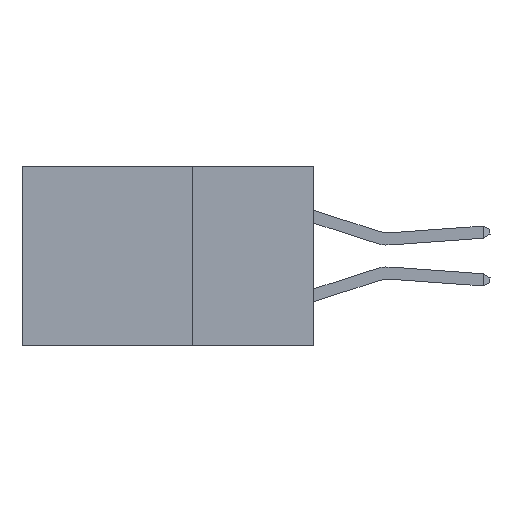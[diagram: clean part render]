
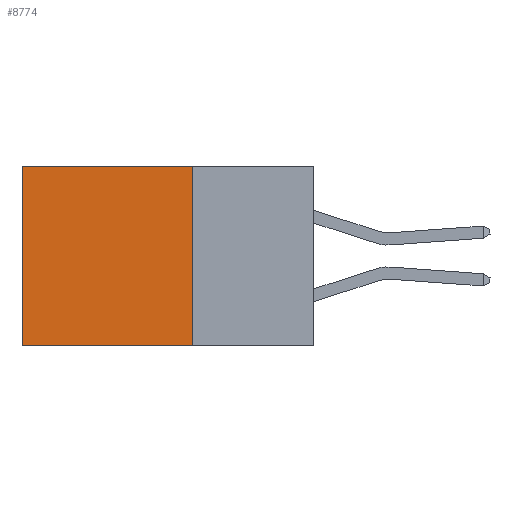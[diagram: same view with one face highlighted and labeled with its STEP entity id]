
A CAD part, left-side view. The second image highlights one B-rep face of the part: STEP entity #8774.
In plain terms, the highlighted planar face has unit normal (-1, 0, 0).
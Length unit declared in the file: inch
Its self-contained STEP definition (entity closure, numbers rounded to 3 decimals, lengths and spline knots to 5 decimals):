
#2572 = VERTEX_POINT ( 'NONE', #25910 ) ;
#3663 = EDGE_CURVE ( 'NONE', #8156, #26611, #4979, .T. ) ;
#4917 = EDGE_LOOP ( 'NONE', ( #30553, #23999, #30525, #23803 ) ) ;
#4979 = LINE ( 'NONE', #27903, #27136 ) ;
#6035 = DIRECTION ( 'NONE',  ( 0., 1., 0. ) ) ;
#6703 = LINE ( 'NONE', #8436, #22310 ) ;
#8019 = VERTEX_POINT ( 'NONE', #17876 ) ;
#8156 = VERTEX_POINT ( 'NONE', #19646 ) ;
#8224 = DIRECTION ( 'NONE',  ( 0., 1., 0. ) ) ;
#8436 = CARTESIAN_POINT ( 'NONE',  ( 0.2875, 0.25, 0. ) ) ;
#8774 = ADVANCED_FACE ( 'NONE', ( #14560 ), #18599, .F. ) ;
#8920 = AXIS2_PLACEMENT_3D ( 'NONE', #31274, #16588, #21604 ) ;
#10647 = VECTOR ( 'NONE', #6035, 39.37008 ) ;
#13384 = DIRECTION ( 'NONE',  ( 0., 0., -1. ) ) ;
#14560 = FACE_OUTER_BOUND ( 'NONE', #4917, .T. ) ;
#15144 = CARTESIAN_POINT ( 'NONE',  ( 0.2875, 0.6, -0.37 ) ) ;
#16588 = DIRECTION ( 'NONE',  ( 1., 0., 0. ) ) ;
#17160 = LINE ( 'NONE', #17858, #10647 ) ;
#17858 = CARTESIAN_POINT ( 'NONE',  ( 0.2875, 0.25, -0.37 ) ) ;
#17876 = CARTESIAN_POINT ( 'NONE',  ( 0.2875, 0.25, -0.37 ) ) ;
#18599 = PLANE ( 'NONE',  #8920 ) ;
#19646 = CARTESIAN_POINT ( 'NONE',  ( 0.2875, 0.6, 0. ) ) ;
#21173 = LINE ( 'NONE', #28477, #26926 ) ;
#21604 = DIRECTION ( 'NONE',  ( 0., 0., -1. ) ) ;
#22310 = VECTOR ( 'NONE', #8224, 39.37008 ) ;
#23092 = DIRECTION ( 'NONE',  ( 0., 0., -1. ) ) ;
#23803 = ORIENTED_EDGE ( 'NONE', *, *, #29656, .T. ) ;
#23999 = ORIENTED_EDGE ( 'NONE', *, *, #24599, .F. ) ;
#24599 = EDGE_CURVE ( 'NONE', #8019, #26611, #17160, .T. ) ;
#25910 = CARTESIAN_POINT ( 'NONE',  ( 0.2875, 0.25, 0. ) ) ;
#26611 = VERTEX_POINT ( 'NONE', #15144 ) ;
#26926 = VECTOR ( 'NONE', #13384, 39.37008 ) ;
#27136 = VECTOR ( 'NONE', #23092, 39.37008 ) ;
#27378 = EDGE_CURVE ( 'NONE', #2572, #8019, #21173, .T. ) ;
#27903 = CARTESIAN_POINT ( 'NONE',  ( 0.2875, 0.6, 0. ) ) ;
#28477 = CARTESIAN_POINT ( 'NONE',  ( 0.2875, 0.25, 0. ) ) ;
#29656 = EDGE_CURVE ( 'NONE', #2572, #8156, #6703, .T. ) ;
#30525 = ORIENTED_EDGE ( 'NONE', *, *, #27378, .F. ) ;
#30553 = ORIENTED_EDGE ( 'NONE', *, *, #3663, .T. ) ;
#31274 = CARTESIAN_POINT ( 'NONE',  ( 0.2875, 0.25, 0. ) ) ;
